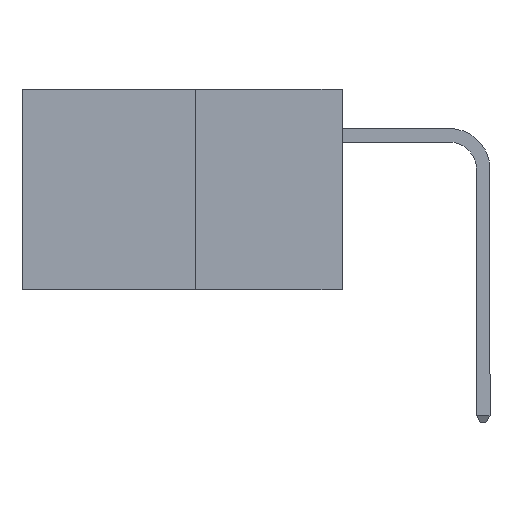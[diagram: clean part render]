
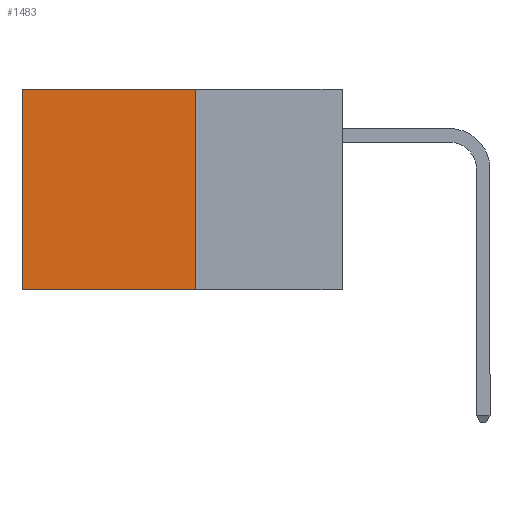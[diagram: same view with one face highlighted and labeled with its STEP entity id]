
A CAD part, left-side view. The second image highlights one B-rep face of the part: STEP entity #1483.
In plain terms, the highlighted planar face has unit normal (-1, 0, 0).
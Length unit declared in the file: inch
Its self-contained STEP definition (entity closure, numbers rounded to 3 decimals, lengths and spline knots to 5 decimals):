
#3 = VERTEX_POINT ( 'NONE', #18422 ) ;
#1483 = ADVANCED_FACE ( 'NONE', ( #13699 ), #26790, .F. ) ;
#1518 = CARTESIAN_POINT ( 'NONE',  ( 0.277, 0.59, -0.37 ) ) ;
#1709 = DIRECTION ( 'NONE',  ( 0., 0., -1. ) ) ;
#2946 = CARTESIAN_POINT ( 'NONE',  ( 0.277, 0.27, -0.37 ) ) ;
#4105 = CARTESIAN_POINT ( 'NONE',  ( 0.277, 0.27, 0. ) ) ;
#4351 = VECTOR ( 'NONE', #24688, 39.37008 ) ;
#4813 = CARTESIAN_POINT ( 'NONE',  ( 0.277, 0.27, -0.37 ) ) ;
#5016 = EDGE_CURVE ( 'NONE', #13711, #3, #7415, .T. ) ;
#5414 = VERTEX_POINT ( 'NONE', #4813 ) ;
#5818 = DIRECTION ( 'NONE',  ( 0., 0., -1. ) ) ;
#6202 = EDGE_CURVE ( 'NONE', #19330, #5414, #26500, .T. ) ;
#7415 = LINE ( 'NONE', #1518, #12574 ) ;
#8583 = LINE ( 'NONE', #18403, #19392 ) ;
#9085 = DIRECTION ( 'NONE',  ( 1., 0., 0. ) ) ;
#9570 = LINE ( 'NONE', #9658, #4351 ) ;
#9658 = CARTESIAN_POINT ( 'NONE',  ( 0.277, 0.27, -0.37 ) ) ;
#11745 = CARTESIAN_POINT ( 'NONE',  ( 0.277, 0.27, -0.37 ) ) ;
#12574 = VECTOR ( 'NONE', #1709, 39.37008 ) ;
#13070 = CARTESIAN_POINT ( 'NONE',  ( 0.277, 0.59, 0. ) ) ;
#13699 = FACE_OUTER_BOUND ( 'NONE', #21694, .T. ) ;
#13711 = VERTEX_POINT ( 'NONE', #13070 ) ;
#14816 = ORIENTED_EDGE ( 'NONE', *, *, #5016, .T. ) ;
#15189 = VECTOR ( 'NONE', #24580, 39.37008 ) ;
#16446 = ORIENTED_EDGE ( 'NONE', *, *, #21810, .F. ) ;
#17953 = ORIENTED_EDGE ( 'NONE', *, *, #25692, .T. ) ;
#18403 = CARTESIAN_POINT ( 'NONE',  ( 0.277, 0.27, 0. ) ) ;
#18422 = CARTESIAN_POINT ( 'NONE',  ( 0.277, 0.59, -0.37 ) ) ;
#18656 = AXIS2_PLACEMENT_3D ( 'NONE', #2946, #9085, #5818 ) ;
#19330 = VERTEX_POINT ( 'NONE', #4105 ) ;
#19392 = VECTOR ( 'NONE', #20561, 39.37008 ) ;
#20561 = DIRECTION ( 'NONE',  ( 0., 1., 0. ) ) ;
#21557 = ORIENTED_EDGE ( 'NONE', *, *, #6202, .F. ) ;
#21694 = EDGE_LOOP ( 'NONE', ( #14816, #16446, #21557, #17953 ) ) ;
#21810 = EDGE_CURVE ( 'NONE', #5414, #3, #9570, .T. ) ;
#24580 = DIRECTION ( 'NONE',  ( 0., 0., -1. ) ) ;
#24688 = DIRECTION ( 'NONE',  ( 0., 1., 0. ) ) ;
#25692 = EDGE_CURVE ( 'NONE', #19330, #13711, #8583, .T. ) ;
#26500 = LINE ( 'NONE', #11745, #15189 ) ;
#26790 = PLANE ( 'NONE',  #18656 ) ;
